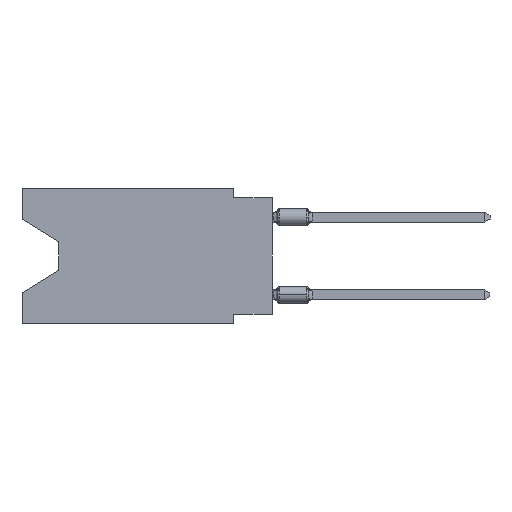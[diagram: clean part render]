
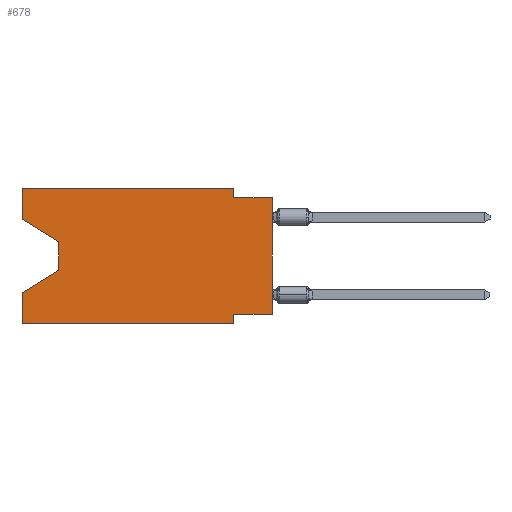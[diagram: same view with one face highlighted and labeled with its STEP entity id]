
A CAD part, left-side view. The second image highlights one B-rep face of the part: STEP entity #678.
In plain terms, the highlighted planar face has unit normal (-1, 0, 0).
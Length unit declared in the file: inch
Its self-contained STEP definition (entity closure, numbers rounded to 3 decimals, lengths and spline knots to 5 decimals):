
#354 = DIRECTION ( 'NONE',  ( 1., 0., 0. ) ) ;
#678 = ADVANCED_FACE ( 'NONE', ( #11363 ), #16849, .F. ) ;
#881 = ORIENTED_EDGE ( 'NONE', *, *, #18374, .T. ) ;
#883 = DIRECTION ( 'NONE',  ( 0., 0., 1. ) ) ;
#923 = CARTESIAN_POINT ( 'NONE',  ( 0., 0.645, -0.35 ) ) ;
#1253 = DIRECTION ( 'NONE',  ( 0., -1., 0. ) ) ;
#1462 = VECTOR ( 'NONE', #8548, 39.37008 ) ;
#1790 = VECTOR ( 'NONE', #10004, 39.37008 ) ;
#2608 = VECTOR ( 'NONE', #9118, 39.37008 ) ;
#2748 = LINE ( 'NONE', #4505, #1790 ) ;
#2928 = LINE ( 'NONE', #13482, #1462 ) ;
#3286 = CARTESIAN_POINT ( 'NONE',  ( 0., 0.1, 0. ) ) ;
#3634 = EDGE_CURVE ( 'NONE', #14194, #4751, #9467, .T. ) ;
#3683 = LINE ( 'NONE', #12599, #15832 ) ;
#3846 = CARTESIAN_POINT ( 'NONE',  ( 0., 0.1, -0.025 ) ) ;
#4387 = LINE ( 'NONE', #19017, #21242 ) ;
#4505 = CARTESIAN_POINT ( 'NONE',  ( 0., 0.55, -0.138 ) ) ;
#4516 = ORIENTED_EDGE ( 'NONE', *, *, #6864, .T. ) ;
#4751 = VERTEX_POINT ( 'NONE', #14315 ) ;
#5118 = VERTEX_POINT ( 'NONE', #7569 ) ;
#5621 = DIRECTION ( 'NONE',  ( 0., -1., 0. ) ) ;
#5847 = CARTESIAN_POINT ( 'NONE',  ( 0., 0.645, -0.26975 ) ) ;
#5940 = LINE ( 'NONE', #20219, #9843 ) ;
#6035 = CARTESIAN_POINT ( 'NONE',  ( 0., 0., -0.325 ) ) ;
#6513 = EDGE_LOOP ( 'NONE', ( #11347, #4516, #14790, #18832, #881, #22458, #12740, #19700, #9345, #10940, #15448, #17167 ) ) ;
#6850 = EDGE_CURVE ( 'NONE', #22859, #22639, #4387, .T. ) ;
#6864 = EDGE_CURVE ( 'NONE', #10830, #15294, #2748, .T. ) ;
#7569 = CARTESIAN_POINT ( 'NONE',  ( 0., 0.1, 0. ) ) ;
#8548 = DIRECTION ( 'NONE',  ( 0., -0.855, -0.519 ) ) ;
#9083 = EDGE_CURVE ( 'NONE', #4751, #9566, #14608, .T. ) ;
#9118 = DIRECTION ( 'NONE',  ( 0., 1., 0. ) ) ;
#9124 = AXIS2_PLACEMENT_3D ( 'NONE', #16387, #354, #14645 ) ;
#9345 = ORIENTED_EDGE ( 'NONE', *, *, #10612, .F. ) ;
#9397 = VERTEX_POINT ( 'NONE', #19146 ) ;
#9467 = LINE ( 'NONE', #16142, #2608 ) ;
#9566 = VERTEX_POINT ( 'NONE', #21942 ) ;
#9843 = VECTOR ( 'NONE', #11334, 39.37008 ) ;
#10004 = DIRECTION ( 'NONE',  ( 0., 0., -1. ) ) ;
#10495 = EDGE_CURVE ( 'NONE', #5118, #13025, #19334, .T. ) ;
#10612 = EDGE_CURVE ( 'NONE', #13025, #15231, #16279, .T. ) ;
#10830 = VERTEX_POINT ( 'NONE', #17443 ) ;
#10940 = ORIENTED_EDGE ( 'NONE', *, *, #10495, .F. ) ;
#10976 = VECTOR ( 'NONE', #1253, 39.37008 ) ;
#11334 = DIRECTION ( 'NONE',  ( 0., 0.855, -0.519 ) ) ;
#11347 = ORIENTED_EDGE ( 'NONE', *, *, #14757, .T. ) ;
#11363 = FACE_OUTER_BOUND ( 'NONE', #6513, .T. ) ;
#11781 = CARTESIAN_POINT ( 'NONE',  ( 0., 0., 0. ) ) ;
#12599 = CARTESIAN_POINT ( 'NONE',  ( 0., 0.645, 0. ) ) ;
#12740 = ORIENTED_EDGE ( 'NONE', *, *, #3634, .F. ) ;
#13025 = VERTEX_POINT ( 'NONE', #3846 ) ;
#13086 = DIRECTION ( 'NONE',  ( 0., 0., -1. ) ) ;
#13482 = CARTESIAN_POINT ( 'NONE',  ( 0., 0.645, -0.08025 ) ) ;
#13544 = LINE ( 'NONE', #16806, #18157 ) ;
#14194 = VERTEX_POINT ( 'NONE', #6035 ) ;
#14266 = VECTOR ( 'NONE', #5621, 39.37008 ) ;
#14315 = CARTESIAN_POINT ( 'NONE',  ( 0., 0.1, -0.325 ) ) ;
#14591 = DIRECTION ( 'NONE',  ( 0., -1., 0. ) ) ;
#14608 = LINE ( 'NONE', #19859, #15701 ) ;
#14645 = DIRECTION ( 'NONE',  ( 0., 0., -1. ) ) ;
#14757 = EDGE_CURVE ( 'NONE', #9397, #10830, #2928, .T. ) ;
#14790 = ORIENTED_EDGE ( 'NONE', *, *, #20031, .T. ) ;
#15231 = VERTEX_POINT ( 'NONE', #19165 ) ;
#15294 = VERTEX_POINT ( 'NONE', #22897 ) ;
#15448 = ORIENTED_EDGE ( 'NONE', *, *, #18496, .F. ) ;
#15548 = CARTESIAN_POINT ( 'NONE',  ( 0., 0.645, 0. ) ) ;
#15701 = VECTOR ( 'NONE', #13086, 39.37008 ) ;
#15832 = VECTOR ( 'NONE', #14591, 39.37008 ) ;
#16142 = CARTESIAN_POINT ( 'NONE',  ( 0., 0., -0.325 ) ) ;
#16245 = VERTEX_POINT ( 'NONE', #15548 ) ;
#16279 = LINE ( 'NONE', #21655, #14266 ) ;
#16387 = CARTESIAN_POINT ( 'NONE',  ( 0., 0.645, 0. ) ) ;
#16806 = CARTESIAN_POINT ( 'NONE',  ( 0., 0.645, 0. ) ) ;
#16849 = PLANE ( 'NONE',  #9124 ) ;
#17167 = ORIENTED_EDGE ( 'NONE', *, *, #22011, .F. ) ;
#17292 = LINE ( 'NONE', #19159, #10976 ) ;
#17443 = CARTESIAN_POINT ( 'NONE',  ( 0., 0.55, -0.138 ) ) ;
#18157 = VECTOR ( 'NONE', #883, 39.37008 ) ;
#18374 = EDGE_CURVE ( 'NONE', #22859, #9566, #17292, .T. ) ;
#18496 = EDGE_CURVE ( 'NONE', #16245, #5118, #3683, .T. ) ;
#18832 = ORIENTED_EDGE ( 'NONE', *, *, #6850, .F. ) ;
#18915 = DIRECTION ( 'NONE',  ( 0., 0., 1. ) ) ;
#19017 = CARTESIAN_POINT ( 'NONE',  ( 0., 0.645, 0. ) ) ;
#19146 = CARTESIAN_POINT ( 'NONE',  ( 0., 0.645, -0.08025 ) ) ;
#19159 = CARTESIAN_POINT ( 'NONE',  ( 0., 0.645, -0.35 ) ) ;
#19165 = CARTESIAN_POINT ( 'NONE',  ( 0., 0., -0.025 ) ) ;
#19271 = VECTOR ( 'NONE', #18915, 39.37008 ) ;
#19334 = LINE ( 'NONE', #3286, #22460 ) ;
#19700 = ORIENTED_EDGE ( 'NONE', *, *, #21943, .T. ) ;
#19859 = CARTESIAN_POINT ( 'NONE',  ( 0., 0.1, -0.35 ) ) ;
#20031 = EDGE_CURVE ( 'NONE', #15294, #22639, #5940, .T. ) ;
#20219 = CARTESIAN_POINT ( 'NONE',  ( 0., 0.55, -0.212 ) ) ;
#21242 = VECTOR ( 'NONE', #22648, 39.37008 ) ;
#21655 = CARTESIAN_POINT ( 'NONE',  ( 0., 0., -0.025 ) ) ;
#21942 = CARTESIAN_POINT ( 'NONE',  ( 0., 0.1, -0.35 ) ) ;
#21943 = EDGE_CURVE ( 'NONE', #14194, #15231, #22305, .T. ) ;
#22011 = EDGE_CURVE ( 'NONE', #9397, #16245, #13544, .T. ) ;
#22305 = LINE ( 'NONE', #11781, #19271 ) ;
#22458 = ORIENTED_EDGE ( 'NONE', *, *, #9083, .F. ) ;
#22460 = VECTOR ( 'NONE', #22840, 39.37008 ) ;
#22639 = VERTEX_POINT ( 'NONE', #5847 ) ;
#22648 = DIRECTION ( 'NONE',  ( 0., 0., 1. ) ) ;
#22840 = DIRECTION ( 'NONE',  ( 0., 0., -1. ) ) ;
#22859 = VERTEX_POINT ( 'NONE', #923 ) ;
#22897 = CARTESIAN_POINT ( 'NONE',  ( 0., 0.55, -0.212 ) ) ;
